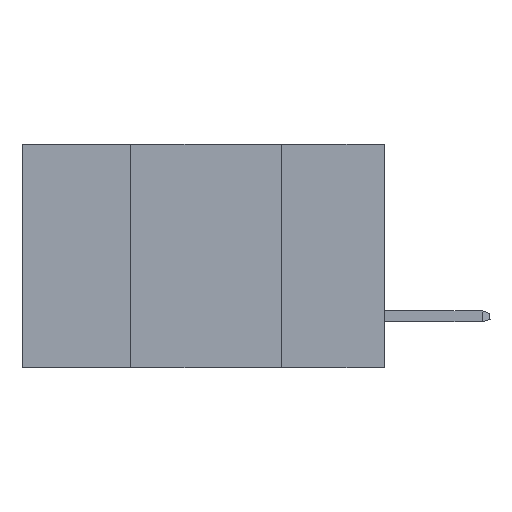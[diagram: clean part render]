
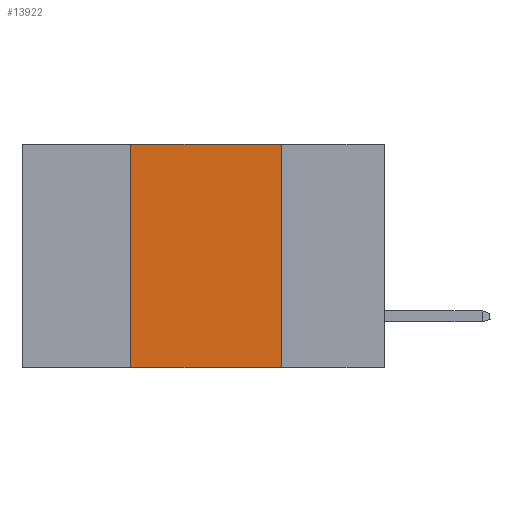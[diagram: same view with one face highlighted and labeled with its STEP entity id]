
A CAD part, left-side view. The second image highlights one B-rep face of the part: STEP entity #13922.
In plain terms, the highlighted planar face has unit normal (-1, 0, 0).
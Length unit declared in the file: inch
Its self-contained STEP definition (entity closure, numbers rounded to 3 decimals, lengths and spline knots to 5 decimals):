
#41 = VERTEX_POINT ( 'NONE', #1186 ) ;
#66 = LINE ( 'NONE', #6586, #14433 ) ;
#803 = EDGE_CURVE ( 'NONE', #2758, #15236, #8379, .T. ) ;
#1143 = DIRECTION ( 'NONE',  ( 0., 0., -1. ) ) ;
#1186 = CARTESIAN_POINT ( 'NONE',  ( 0., 0.17, 0. ) ) ;
#1350 = ORIENTED_EDGE ( 'NONE', *, *, #803, .F. ) ;
#1700 = ORIENTED_EDGE ( 'NONE', *, *, #5930, .F. ) ;
#1856 = DIRECTION ( 'NONE',  ( 0., -1., 0. ) ) ;
#2099 = ORIENTED_EDGE ( 'NONE', *, *, #10282, .T. ) ;
#2242 = ORIENTED_EDGE ( 'NONE', *, *, #14038, .F. ) ;
#2313 = PLANE ( 'NONE',  #15286 ) ;
#2758 = VERTEX_POINT ( 'NONE', #9029 ) ;
#3684 = CARTESIAN_POINT ( 'NONE',  ( 0., 0.42, 0. ) ) ;
#3935 = VECTOR ( 'NONE', #12744, 39.37008 ) ;
#4314 = VECTOR ( 'NONE', #1143, 39.37008 ) ;
#4318 = LINE ( 'NONE', #9327, #3935 ) ;
#5177 = VECTOR ( 'NONE', #5991, 39.37008 ) ;
#5930 = EDGE_CURVE ( 'NONE', #15236, #41, #4318, .T. ) ;
#5991 = DIRECTION ( 'NONE',  ( 0., 0., 1. ) ) ;
#6031 = CARTESIAN_POINT ( 'NONE',  ( 0., 0.6, 0. ) ) ;
#6202 = FACE_OUTER_BOUND ( 'NONE', #14951, .T. ) ;
#6571 = LINE ( 'NONE', #10780, #4314 ) ;
#6586 = CARTESIAN_POINT ( 'NONE',  ( 0., 0.6, -0.37 ) ) ;
#7231 = DIRECTION ( 'NONE',  ( 0., 0., -1. ) ) ;
#8379 = LINE ( 'NONE', #3684, #5177 ) ;
#9029 = CARTESIAN_POINT ( 'NONE',  ( 0., 0.42, -0.37 ) ) ;
#9327 = CARTESIAN_POINT ( 'NONE',  ( 0., 0.6, 0. ) ) ;
#10131 = CARTESIAN_POINT ( 'NONE',  ( 0., 0.42, 0. ) ) ;
#10282 = EDGE_CURVE ( 'NONE', #2758, #14505, #66, .T. ) ;
#10668 = DIRECTION ( 'NONE',  ( 1., 0., 0. ) ) ;
#10780 = CARTESIAN_POINT ( 'NONE',  ( 0., 0.17, 0. ) ) ;
#12744 = DIRECTION ( 'NONE',  ( 0., -1., 0. ) ) ;
#13922 = ADVANCED_FACE ( 'NONE', ( #6202 ), #2313, .F. ) ;
#14038 = EDGE_CURVE ( 'NONE', #41, #14505, #6571, .T. ) ;
#14433 = VECTOR ( 'NONE', #1856, 39.37008 ) ;
#14505 = VERTEX_POINT ( 'NONE', #15376 ) ;
#14951 = EDGE_LOOP ( 'NONE', ( #2242, #1700, #1350, #2099 ) ) ;
#15236 = VERTEX_POINT ( 'NONE', #10131 ) ;
#15286 = AXIS2_PLACEMENT_3D ( 'NONE', #6031, #10668, #7231 ) ;
#15376 = CARTESIAN_POINT ( 'NONE',  ( 0., 0.17, -0.37 ) ) ;
